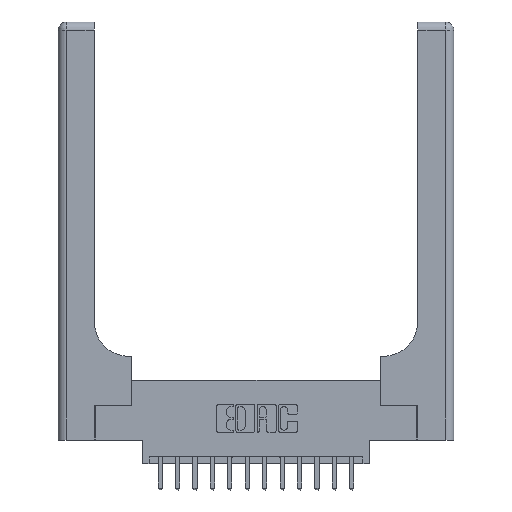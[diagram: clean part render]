
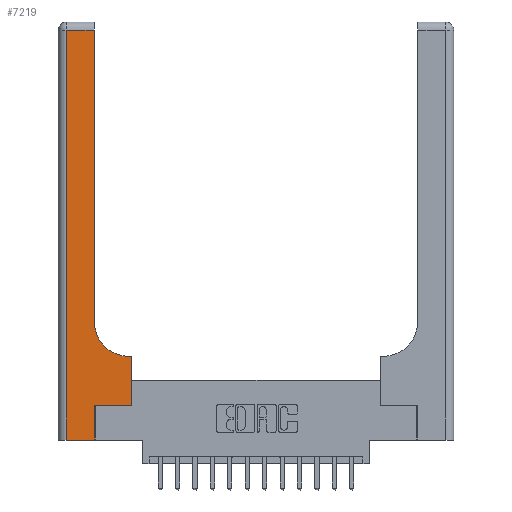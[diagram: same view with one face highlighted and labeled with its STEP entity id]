
A CAD part, top view. The second image highlights one B-rep face of the part: STEP entity #7219.
In plain terms, the highlighted planar face has unit normal (0, 0, 1).
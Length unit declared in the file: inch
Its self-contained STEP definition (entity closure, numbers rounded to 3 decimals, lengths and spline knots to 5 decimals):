
#590 = CARTESIAN_POINT ( 'NONE',  ( 0.26, 2.94, 0.37 ) ) ;
#675 = DIRECTION ( 'NONE',  ( 0., 1., 0. ) ) ;
#699 = DIRECTION ( 'NONE',  ( -1., 0., 0. ) ) ;
#718 = VERTEX_POINT ( 'NONE', #9982 ) ;
#1002 = VERTEX_POINT ( 'NONE', #2149 ) ;
#1355 = CARTESIAN_POINT ( 'NONE',  ( 0.265, 0.25, 0.37 ) ) ;
#1357 = ORIENTED_EDGE ( 'NONE', *, *, #13234, .T. ) ;
#1513 = LINE ( 'NONE', #13855, #9183 ) ;
#1924 = VECTOR ( 'NONE', #675, 39.37008 ) ;
#1939 = EDGE_CURVE ( 'NONE', #16556, #13647, #5060, .T. ) ;
#2011 = ORIENTED_EDGE ( 'NONE', *, *, #3317, .T. ) ;
#2096 = VECTOR ( 'NONE', #12670, 39.37008 ) ;
#2149 = CARTESIAN_POINT ( 'NONE',  ( 0.51, 0.6, 0.37 ) ) ;
#2382 = VERTEX_POINT ( 'NONE', #4256 ) ;
#2695 = LINE ( 'NONE', #1355, #13638 ) ;
#2728 = VERTEX_POINT ( 'NONE', #10665 ) ;
#3035 = LINE ( 'NONE', #9748, #16926 ) ;
#3314 = DIRECTION ( 'NONE',  ( 0., 0., -1. ) ) ;
#3317 = EDGE_CURVE ( 'NONE', #10138, #2728, #11237, .T. ) ;
#3466 = CARTESIAN_POINT ( 'NONE',  ( 0.26, 0.85, 0.37 ) ) ;
#3490 = FACE_OUTER_BOUND ( 'NONE', #9727, .T. ) ;
#3572 = ORIENTED_EDGE ( 'NONE', *, *, #7513, .T. ) ;
#3895 = VERTEX_POINT ( 'NONE', #4523 ) ;
#4256 = CARTESIAN_POINT ( 'NONE',  ( 0.06, 2.94, 0.37 ) ) ;
#4523 = CARTESIAN_POINT ( 'NONE',  ( 0.528, 0.6, 0.37 ) ) ;
#4598 = CARTESIAN_POINT ( 'NONE',  ( 0.51, 0.85, 0.37 ) ) ;
#4700 = CARTESIAN_POINT ( 'NONE',  ( 0.26, 3., 0.37 ) ) ;
#5060 = LINE ( 'NONE', #4700, #1924 ) ;
#5213 = CARTESIAN_POINT ( 'NONE',  ( 0.265, 0., 0.37 ) ) ;
#5548 = CARTESIAN_POINT ( 'NONE',  ( 0., 2.94, 0.37 ) ) ;
#5631 = DIRECTION ( 'NONE',  ( -1., 0., 0. ) ) ;
#5755 = VECTOR ( 'NONE', #16717, 39.37008 ) ;
#6282 = PLANE ( 'NONE',  #16500 ) ;
#6399 = EDGE_CURVE ( 'NONE', #14841, #3895, #15548, .T. ) ;
#6493 = VECTOR ( 'NONE', #10732, 39.37008 ) ;
#6994 = EDGE_CURVE ( 'NONE', #13647, #2382, #15364, .T. ) ;
#7219 = ADVANCED_FACE ( 'NONE', ( #3490 ), #6282, .F. ) ;
#7513 = EDGE_CURVE ( 'NONE', #1002, #16556, #15338, .T. ) ;
#7608 = AXIS2_PLACEMENT_3D ( 'NONE', #4598, #10154, #8803 ) ;
#8177 = EDGE_CURVE ( 'NONE', #718, #14841, #2695, .T. ) ;
#8269 = CARTESIAN_POINT ( 'NONE',  ( 0., 0., 0.37 ) ) ;
#8803 = DIRECTION ( 'NONE',  ( 1., 0., 0. ) ) ;
#8881 = ORIENTED_EDGE ( 'NONE', *, *, #6994, .T. ) ;
#9119 = CARTESIAN_POINT ( 'NONE',  ( 0., 3., 0.37 ) ) ;
#9183 = VECTOR ( 'NONE', #5631, 39.37008 ) ;
#9727 = EDGE_LOOP ( 'NONE', ( #11731, #8881, #16698, #2011, #11961, #12183, #15131, #1357, #3572 ) ) ;
#9748 = CARTESIAN_POINT ( 'NONE',  ( 0.06, 3., 0.37 ) ) ;
#9982 = CARTESIAN_POINT ( 'NONE',  ( 0.265, 0.25, 0.37 ) ) ;
#10138 = VERTEX_POINT ( 'NONE', #11040 ) ;
#10154 = DIRECTION ( 'NONE',  ( 0., 0., -1. ) ) ;
#10665 = CARTESIAN_POINT ( 'NONE',  ( 0.265, 0., 0.37 ) ) ;
#10732 = DIRECTION ( 'NONE',  ( 0., 1., 0. ) ) ;
#11040 = CARTESIAN_POINT ( 'NONE',  ( 0.06, 0., 0.37 ) ) ;
#11050 = VECTOR ( 'NONE', #12578, 39.37008 ) ;
#11159 = CARTESIAN_POINT ( 'NONE',  ( 0.528, 0.25, 0.37 ) ) ;
#11237 = LINE ( 'NONE', #8269, #5755 ) ;
#11422 = EDGE_CURVE ( 'NONE', #2728, #718, #17539, .T. ) ;
#11731 = ORIENTED_EDGE ( 'NONE', *, *, #1939, .T. ) ;
#11961 = ORIENTED_EDGE ( 'NONE', *, *, #11422, .T. ) ;
#12183 = ORIENTED_EDGE ( 'NONE', *, *, #8177, .T. ) ;
#12578 = DIRECTION ( 'NONE',  ( -1., 0., 0. ) ) ;
#12668 = CARTESIAN_POINT ( 'NONE',  ( 0.528, 0.25, 0.37 ) ) ;
#12670 = DIRECTION ( 'NONE',  ( 0., 1., 0. ) ) ;
#13234 = EDGE_CURVE ( 'NONE', #3895, #1002, #1513, .T. ) ;
#13638 = VECTOR ( 'NONE', #15014, 39.37008 ) ;
#13647 = VERTEX_POINT ( 'NONE', #590 ) ;
#13855 = CARTESIAN_POINT ( 'NONE',  ( 0.26, 0.6, 0.37 ) ) ;
#14021 = DIRECTION ( 'NONE',  ( 0., -1., 0. ) ) ;
#14841 = VERTEX_POINT ( 'NONE', #12668 ) ;
#14861 = EDGE_CURVE ( 'NONE', #2382, #10138, #3035, .T. ) ;
#15014 = DIRECTION ( 'NONE',  ( 1., 0., 0. ) ) ;
#15131 = ORIENTED_EDGE ( 'NONE', *, *, #6399, .T. ) ;
#15338 = CIRCLE ( 'NONE', #7608, 0.25 ) ;
#15364 = LINE ( 'NONE', #5548, #11050 ) ;
#15548 = LINE ( 'NONE', #11159, #2096 ) ;
#16500 = AXIS2_PLACEMENT_3D ( 'NONE', #9119, #3314, #699 ) ;
#16556 = VERTEX_POINT ( 'NONE', #3466 ) ;
#16698 = ORIENTED_EDGE ( 'NONE', *, *, #14861, .T. ) ;
#16717 = DIRECTION ( 'NONE',  ( 1., 0., 0. ) ) ;
#16926 = VECTOR ( 'NONE', #14021, 39.37008 ) ;
#17539 = LINE ( 'NONE', #5213, #6493 ) ;
